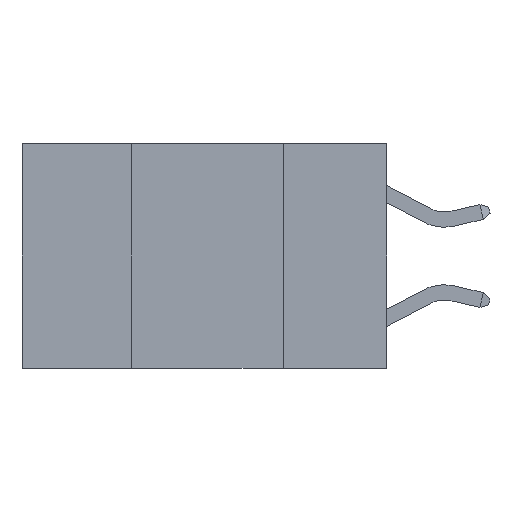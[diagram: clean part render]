
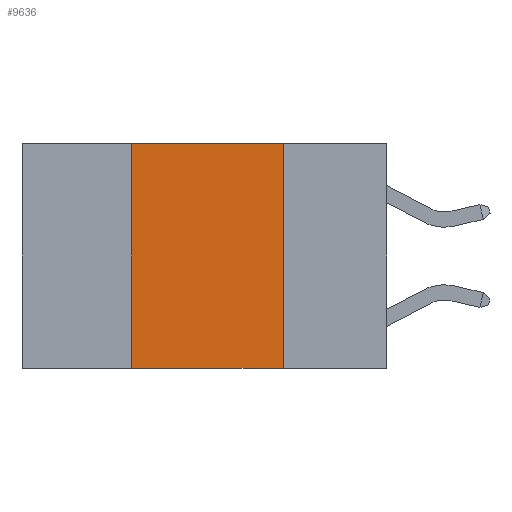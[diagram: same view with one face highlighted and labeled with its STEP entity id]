
A CAD part, left-side view. The second image highlights one B-rep face of the part: STEP entity #9636.
In plain terms, the highlighted planar face has unit normal (-1, 0, 0).
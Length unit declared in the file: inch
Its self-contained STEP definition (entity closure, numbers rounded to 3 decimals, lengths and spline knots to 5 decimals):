
#485 = CARTESIAN_POINT ( 'NONE',  ( 0., 0.17, 0. ) ) ;
#1335 = PLANE ( 'NONE',  #14090 ) ;
#1486 = CARTESIAN_POINT ( 'NONE',  ( 0., 0.42, -0.37 ) ) ;
#2085 = ORIENTED_EDGE ( 'NONE', *, *, #3724, .T. ) ;
#2234 = ORIENTED_EDGE ( 'NONE', *, *, #12003, .F. ) ;
#2952 = DIRECTION ( 'NONE',  ( 0., -1., 0. ) ) ;
#3087 = CARTESIAN_POINT ( 'NONE',  ( 0., 0.17, 0. ) ) ;
#3250 = CARTESIAN_POINT ( 'NONE',  ( 0., 0.42, 0. ) ) ;
#3336 = DIRECTION ( 'NONE',  ( 0., 0., -1. ) ) ;
#3724 = EDGE_CURVE ( 'NONE', #17059, #16562, #11284, .T. ) ;
#3911 = LINE ( 'NONE', #485, #9986 ) ;
#3926 = VECTOR ( 'NONE', #9665, 39.37008 ) ;
#5728 = CARTESIAN_POINT ( 'NONE',  ( 0., 0.6, 0. ) ) ;
#5829 = CARTESIAN_POINT ( 'NONE',  ( 0., 0.42, 0. ) ) ;
#7217 = DIRECTION ( 'NONE',  ( 0., 0., -1. ) ) ;
#7890 = EDGE_LOOP ( 'NONE', ( #12888, #2234, #17241, #2085 ) ) ;
#8184 = FACE_OUTER_BOUND ( 'NONE', #7890, .T. ) ;
#9590 = VECTOR ( 'NONE', #2952, 39.37008 ) ;
#9636 = ADVANCED_FACE ( 'NONE', ( #8184 ), #1335, .F. ) ;
#9665 = DIRECTION ( 'NONE',  ( 0., -1., 0. ) ) ;
#9986 = VECTOR ( 'NONE', #3336, 39.37008 ) ;
#10315 = EDGE_CURVE ( 'NONE', #17059, #14659, #15278, .T. ) ;
#11284 = LINE ( 'NONE', #13758, #3926 ) ;
#11614 = VECTOR ( 'NONE', #12755, 39.37008 ) ;
#12003 = EDGE_CURVE ( 'NONE', #14659, #13462, #17727, .T. ) ;
#12755 = DIRECTION ( 'NONE',  ( 0., 0., 1. ) ) ;
#12888 = ORIENTED_EDGE ( 'NONE', *, *, #13591, .F. ) ;
#13462 = VERTEX_POINT ( 'NONE', #3087 ) ;
#13591 = EDGE_CURVE ( 'NONE', #13462, #16562, #3911, .T. ) ;
#13758 = CARTESIAN_POINT ( 'NONE',  ( 0., 0.6, -0.37 ) ) ;
#13870 = CARTESIAN_POINT ( 'NONE',  ( 0., 0.6, 0. ) ) ;
#14090 = AXIS2_PLACEMENT_3D ( 'NONE', #13870, #15486, #7217 ) ;
#14659 = VERTEX_POINT ( 'NONE', #3250 ) ;
#15278 = LINE ( 'NONE', #5829, #11614 ) ;
#15486 = DIRECTION ( 'NONE',  ( 1., 0., 0. ) ) ;
#15768 = CARTESIAN_POINT ( 'NONE',  ( 0., 0.17, -0.37 ) ) ;
#16562 = VERTEX_POINT ( 'NONE', #15768 ) ;
#17059 = VERTEX_POINT ( 'NONE', #1486 ) ;
#17241 = ORIENTED_EDGE ( 'NONE', *, *, #10315, .F. ) ;
#17727 = LINE ( 'NONE', #5728, #9590 ) ;
